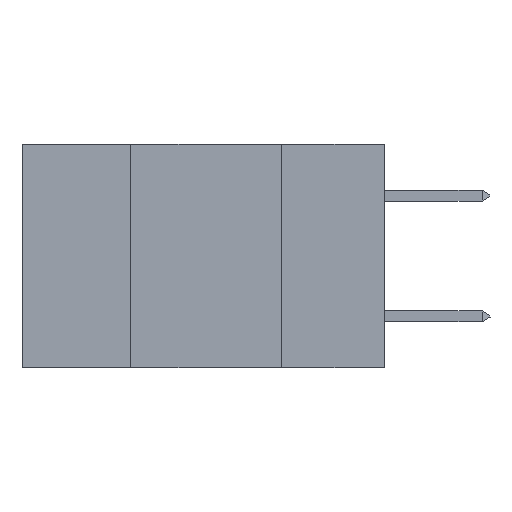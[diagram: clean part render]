
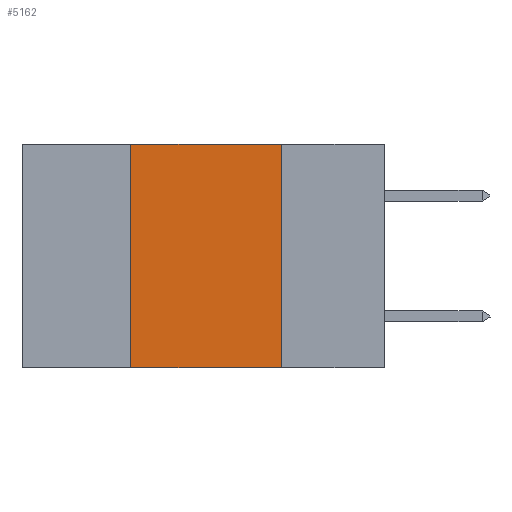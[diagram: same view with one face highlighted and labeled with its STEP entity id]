
A CAD part, left-side view. The second image highlights one B-rep face of the part: STEP entity #5162.
In plain terms, the highlighted planar face has unit normal (-1, 0, 0).
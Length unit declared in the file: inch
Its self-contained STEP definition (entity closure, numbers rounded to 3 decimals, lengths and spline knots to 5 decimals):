
#20 = ORIENTED_EDGE ( 'NONE', *, *, #10135, .F. ) ;
#952 = VERTEX_POINT ( 'NONE', #6315 ) ;
#1487 = LINE ( 'NONE', #5024, #13391 ) ;
#2007 = DIRECTION ( 'NONE',  ( 0., 0., -1. ) ) ;
#2046 = CARTESIAN_POINT ( 'NONE',  ( 0., 0.6, 0. ) ) ;
#3298 = EDGE_LOOP ( 'NONE', ( #15473, #20, #31145, #31256 ) ) ;
#4342 = EDGE_CURVE ( 'NONE', #7469, #27718, #41026, .T. ) ;
#4836 = LINE ( 'NONE', #2046, #30086 ) ;
#5024 = CARTESIAN_POINT ( 'NONE',  ( 0., 0.42, 0. ) ) ;
#5105 = AXIS2_PLACEMENT_3D ( 'NONE', #8225, #17926, #11576 ) ;
#5162 = ADVANCED_FACE ( 'NONE', ( #35730 ), #34706, .F. ) ;
#6315 = CARTESIAN_POINT ( 'NONE',  ( 0., 0.42, 0. ) ) ;
#6558 = CARTESIAN_POINT ( 'NONE',  ( 0., 0.17, 0. ) ) ;
#6971 = CARTESIAN_POINT ( 'NONE',  ( 0., 0.17, -0.37 ) ) ;
#7469 = VERTEX_POINT ( 'NONE', #38177 ) ;
#8225 = CARTESIAN_POINT ( 'NONE',  ( 0., 0.6, 0. ) ) ;
#10135 = EDGE_CURVE ( 'NONE', #952, #39806, #4836, .T. ) ;
#11495 = VECTOR ( 'NONE', #18862, 39.37008 ) ;
#11576 = DIRECTION ( 'NONE',  ( 0., 0., -1. ) ) ;
#13391 = VECTOR ( 'NONE', #15148, 39.37008 ) ;
#15148 = DIRECTION ( 'NONE',  ( 0., 0., 1. ) ) ;
#15473 = ORIENTED_EDGE ( 'NONE', *, *, #21460, .F. ) ;
#17926 = DIRECTION ( 'NONE',  ( 1., 0., 0. ) ) ;
#18862 = DIRECTION ( 'NONE',  ( 0., -1., 0. ) ) ;
#21460 = EDGE_CURVE ( 'NONE', #39806, #27718, #27428, .T. ) ;
#21850 = CARTESIAN_POINT ( 'NONE',  ( 0., 0.17, 0. ) ) ;
#22020 = DIRECTION ( 'NONE',  ( 0., -1., 0. ) ) ;
#22152 = EDGE_CURVE ( 'NONE', #7469, #952, #1487, .T. ) ;
#27428 = LINE ( 'NONE', #21850, #35134 ) ;
#27718 = VERTEX_POINT ( 'NONE', #6971 ) ;
#30086 = VECTOR ( 'NONE', #22020, 39.37008 ) ;
#31145 = ORIENTED_EDGE ( 'NONE', *, *, #22152, .F. ) ;
#31256 = ORIENTED_EDGE ( 'NONE', *, *, #4342, .T. ) ;
#32180 = CARTESIAN_POINT ( 'NONE',  ( 0., 0.6, -0.37 ) ) ;
#34706 = PLANE ( 'NONE',  #5105 ) ;
#35134 = VECTOR ( 'NONE', #2007, 39.37008 ) ;
#35730 = FACE_OUTER_BOUND ( 'NONE', #3298, .T. ) ;
#38177 = CARTESIAN_POINT ( 'NONE',  ( 0., 0.42, -0.37 ) ) ;
#39806 = VERTEX_POINT ( 'NONE', #6558 ) ;
#41026 = LINE ( 'NONE', #32180, #11495 ) ;
